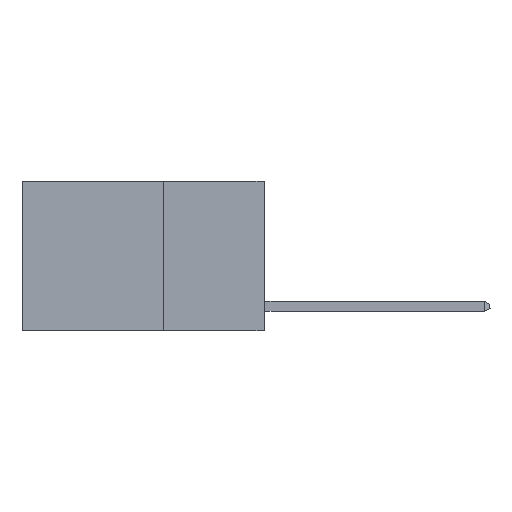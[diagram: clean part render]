
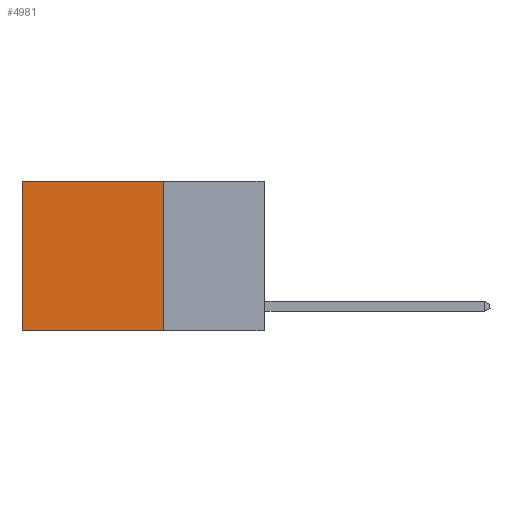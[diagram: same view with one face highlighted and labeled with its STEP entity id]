
A CAD part, left-side view. The second image highlights one B-rep face of the part: STEP entity #4981.
In plain terms, the highlighted planar face has unit normal (-1, 0, 0).
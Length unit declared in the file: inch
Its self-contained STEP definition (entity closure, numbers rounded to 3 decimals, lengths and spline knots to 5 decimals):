
#42 = DIRECTION ( 'NONE',  ( 0., 1., 0. ) ) ;
#1019 = CARTESIAN_POINT ( 'NONE',  ( 0.2625, 0.6, 0. ) ) ;
#1031 = DIRECTION ( 'NONE',  ( 0., 0., -1. ) ) ;
#2318 = LINE ( 'NONE', #12564, #11526 ) ;
#2736 = LINE ( 'NONE', #10553, #5532 ) ;
#3153 = EDGE_LOOP ( 'NONE', ( #5322, #7741, #10404, #7780 ) ) ;
#4369 = CARTESIAN_POINT ( 'NONE',  ( 0.2625, 0.25, 0. ) ) ;
#4981 = ADVANCED_FACE ( 'NONE', ( #16030 ), #5455, .F. ) ;
#5322 = ORIENTED_EDGE ( 'NONE', *, *, #11036, .T. ) ;
#5455 = PLANE ( 'NONE',  #5513 ) ;
#5513 = AXIS2_PLACEMENT_3D ( 'NONE', #4369, #14588, #10918 ) ;
#5532 = VECTOR ( 'NONE', #42, 39.37008 ) ;
#5592 = EDGE_CURVE ( 'NONE', #10750, #16537, #8596, .T. ) ;
#6856 = CARTESIAN_POINT ( 'NONE',  ( 0.2625, 0.6, -0.37 ) ) ;
#7338 = CARTESIAN_POINT ( 'NONE',  ( 0.2625, 0.25, 0. ) ) ;
#7741 = ORIENTED_EDGE ( 'NONE', *, *, #8580, .F. ) ;
#7780 = ORIENTED_EDGE ( 'NONE', *, *, #13696, .T. ) ;
#8580 = EDGE_CURVE ( 'NONE', #16537, #13096, #2736, .T. ) ;
#8596 = LINE ( 'NONE', #7338, #15181 ) ;
#9115 = VERTEX_POINT ( 'NONE', #12958 ) ;
#10404 = ORIENTED_EDGE ( 'NONE', *, *, #5592, .F. ) ;
#10553 = CARTESIAN_POINT ( 'NONE',  ( 0.2625, 0.25, -0.37 ) ) ;
#10750 = VERTEX_POINT ( 'NONE', #16469 ) ;
#10918 = DIRECTION ( 'NONE',  ( 0., 0., -1. ) ) ;
#11036 = EDGE_CURVE ( 'NONE', #9115, #13096, #12789, .T. ) ;
#11233 = VECTOR ( 'NONE', #11515, 39.37008 ) ;
#11515 = DIRECTION ( 'NONE',  ( 0., 0., -1. ) ) ;
#11526 = VECTOR ( 'NONE', #16420, 39.37008 ) ;
#12564 = CARTESIAN_POINT ( 'NONE',  ( 0.2625, 0.25, 0. ) ) ;
#12789 = LINE ( 'NONE', #1019, #11233 ) ;
#12958 = CARTESIAN_POINT ( 'NONE',  ( 0.2625, 0.6, 0. ) ) ;
#13096 = VERTEX_POINT ( 'NONE', #6856 ) ;
#13696 = EDGE_CURVE ( 'NONE', #10750, #9115, #2318, .T. ) ;
#14588 = DIRECTION ( 'NONE',  ( 1., 0., 0. ) ) ;
#15181 = VECTOR ( 'NONE', #1031, 39.37008 ) ;
#16030 = FACE_OUTER_BOUND ( 'NONE', #3153, .T. ) ;
#16149 = CARTESIAN_POINT ( 'NONE',  ( 0.2625, 0.25, -0.37 ) ) ;
#16420 = DIRECTION ( 'NONE',  ( 0., 1., 0. ) ) ;
#16469 = CARTESIAN_POINT ( 'NONE',  ( 0.2625, 0.25, 0. ) ) ;
#16537 = VERTEX_POINT ( 'NONE', #16149 ) ;
